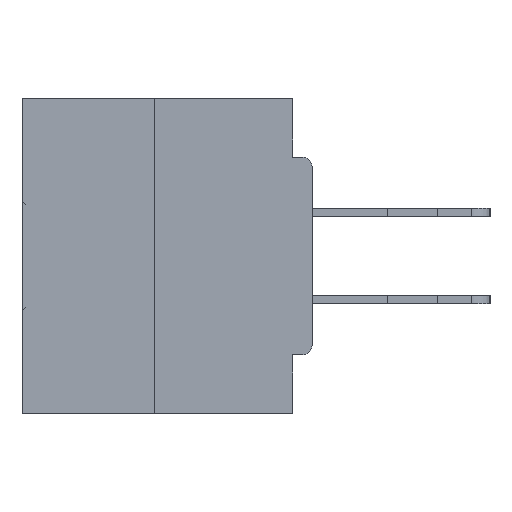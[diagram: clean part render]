
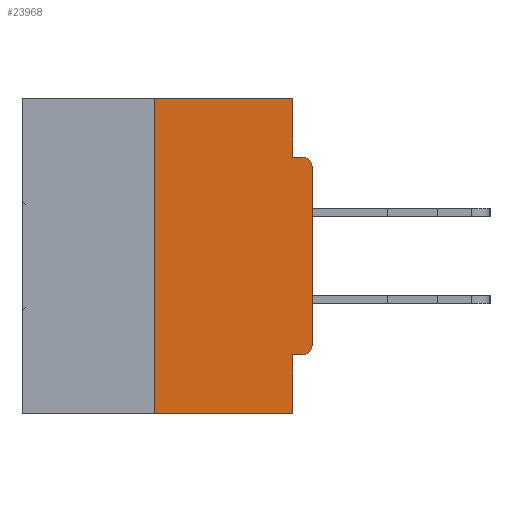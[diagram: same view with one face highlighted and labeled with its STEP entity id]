
A CAD part, left-side view. The second image highlights one B-rep face of the part: STEP entity #23968.
In plain terms, the highlighted planar face has unit normal (-1, 0, 0).
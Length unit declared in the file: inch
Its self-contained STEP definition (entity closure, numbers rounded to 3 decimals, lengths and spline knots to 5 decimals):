
#70 = CARTESIAN_POINT ( 'NONE',  ( 0., 0.015, -0.1085 ) ) ;
#123 = LINE ( 'NONE', #26899, #35440 ) ;
#1087 = VERTEX_POINT ( 'NONE', #8776 ) ;
#1341 = ORIENTED_EDGE ( 'NONE', *, *, #15577, .F. ) ;
#2043 = LINE ( 'NONE', #12261, #20298 ) ;
#2280 = EDGE_CURVE ( 'NONE', #7805, #30325, #18737, .T. ) ;
#2711 = DIRECTION ( 'NONE',  ( 0., 0., 1. ) ) ;
#2891 = LINE ( 'NONE', #3313, #11492 ) ;
#3052 = EDGE_CURVE ( 'NONE', #33925, #22421, #33907, .T. ) ;
#3313 = CARTESIAN_POINT ( 'NONE',  ( 0., 0.46, 0. ) ) ;
#4376 = VECTOR ( 'NONE', #14509, 39.37008 ) ;
#4506 = CARTESIAN_POINT ( 'NONE',  ( 0., 0.25, 0. ) ) ;
#5059 = EDGE_CURVE ( 'NONE', #30719, #29410, #36116, .T. ) ;
#5201 = VECTOR ( 'NONE', #11336, 39.37008 ) ;
#6873 = CARTESIAN_POINT ( 'NONE',  ( 0., 0.015, -0.0935 ) ) ;
#7344 = ORIENTED_EDGE ( 'NONE', *, *, #41202, .F. ) ;
#7805 = VERTEX_POINT ( 'NONE', #12624 ) ;
#8361 = DIRECTION ( 'NONE',  ( 0., 0., -1. ) ) ;
#8721 = CARTESIAN_POINT ( 'NONE',  ( 0., 0., -0.0935 ) ) ;
#8776 = CARTESIAN_POINT ( 'NONE',  ( 0., 0.031, 0. ) ) ;
#9015 = DIRECTION ( 'NONE',  ( -1., 0., 0. ) ) ;
#9055 = CARTESIAN_POINT ( 'NONE',  ( 0., 0., -0.1085 ) ) ;
#9885 = ORIENTED_EDGE ( 'NONE', *, *, #34799, .T. ) ;
#10017 = VERTEX_POINT ( 'NONE', #4506 ) ;
#10752 = VERTEX_POINT ( 'NONE', #9055 ) ;
#11336 = DIRECTION ( 'NONE',  ( 0., -1., 0. ) ) ;
#11492 = VECTOR ( 'NONE', #39909, 39.37008 ) ;
#11627 = DIRECTION ( 'NONE',  ( -1., 0., 0. ) ) ;
#12080 = CARTESIAN_POINT ( 'NONE',  ( 0., 0.25, 0. ) ) ;
#12261 = CARTESIAN_POINT ( 'NONE',  ( 0., 0., -0.4065 ) ) ;
#12624 = CARTESIAN_POINT ( 'NONE',  ( 0., 0.031, -0.0935 ) ) ;
#12968 = DIRECTION ( 'NONE',  ( 0., 0., -1. ) ) ;
#13441 = ORIENTED_EDGE ( 'NONE', *, *, #5059, .T. ) ;
#13727 = EDGE_CURVE ( 'NONE', #41756, #29410, #24661, .T. ) ;
#14509 = DIRECTION ( 'NONE',  ( 0., 0., 1. ) ) ;
#14724 = CARTESIAN_POINT ( 'NONE',  ( 0., 0., 0. ) ) ;
#14900 = CARTESIAN_POINT ( 'NONE',  ( 0., 0.015, -0.3915 ) ) ;
#15320 = DIRECTION ( 'NONE',  ( 0., 1., 0. ) ) ;
#15577 = EDGE_CURVE ( 'NONE', #1087, #7805, #123, .T. ) ;
#16372 = CARTESIAN_POINT ( 'NONE',  ( 0., 0.031, -0.4065 ) ) ;
#16711 = LINE ( 'NONE', #14724, #4376 ) ;
#16902 = AXIS2_PLACEMENT_3D ( 'NONE', #70, #9015, #30112 ) ;
#17623 = EDGE_CURVE ( 'NONE', #10752, #30325, #25954, .T. ) ;
#17891 = ORIENTED_EDGE ( 'NONE', *, *, #13727, .F. ) ;
#18737 = LINE ( 'NONE', #8721, #5201 ) ;
#19232 = ORIENTED_EDGE ( 'NONE', *, *, #3052, .T. ) ;
#19343 = EDGE_CURVE ( 'NONE', #10017, #1087, #2891, .T. ) ;
#20298 = VECTOR ( 'NONE', #15320, 39.37008 ) ;
#21587 = FACE_OUTER_BOUND ( 'NONE', #33584, .T. ) ;
#21800 = DIRECTION ( 'NONE',  ( 0., 0., -1. ) ) ;
#22421 = VERTEX_POINT ( 'NONE', #42046 ) ;
#22875 = CARTESIAN_POINT ( 'NONE',  ( 0., 0.46, 0. ) ) ;
#23968 = ADVANCED_FACE ( 'NONE', ( #21587 ), #32689, .F. ) ;
#24661 = LINE ( 'NONE', #37962, #29451 ) ;
#25738 = DIRECTION ( 'NONE',  ( 1., 0., 0. ) ) ;
#25954 = CIRCLE ( 'NONE', #16902, 0.015 ) ;
#26320 = DIRECTION ( 'NONE',  ( 0., -1., 0. ) ) ;
#26899 = CARTESIAN_POINT ( 'NONE',  ( 0., 0.031, 0. ) ) ;
#27464 = VECTOR ( 'NONE', #2711, 39.37008 ) ;
#27690 = CARTESIAN_POINT ( 'NONE',  ( 0., 0.25, -0.5 ) ) ;
#27930 = AXIS2_PLACEMENT_3D ( 'NONE', #22875, #25738, #35752 ) ;
#29062 = LINE ( 'NONE', #12080, #27464 ) ;
#29410 = VERTEX_POINT ( 'NONE', #32285 ) ;
#29451 = VECTOR ( 'NONE', #21800, 39.37008 ) ;
#29796 = CARTESIAN_POINT ( 'NONE',  ( 0., 0.46, -0.5 ) ) ;
#30112 = DIRECTION ( 'NONE',  ( 0., 0., -1. ) ) ;
#30140 = CARTESIAN_POINT ( 'NONE',  ( 0., 0.015, -0.4065 ) ) ;
#30325 = VERTEX_POINT ( 'NONE', #6873 ) ;
#30719 = VERTEX_POINT ( 'NONE', #27690 ) ;
#32127 = VECTOR ( 'NONE', #26320, 39.37008 ) ;
#32285 = CARTESIAN_POINT ( 'NONE',  ( 0., 0.031, -0.5 ) ) ;
#32422 = ORIENTED_EDGE ( 'NONE', *, *, #17623, .T. ) ;
#32689 = PLANE ( 'NONE',  #27930 ) ;
#33584 = EDGE_LOOP ( 'NONE', ( #41730, #7344, #13441, #17891, #38287, #19232, #9885, #32422, #39816, #1341 ) ) ;
#33907 = CIRCLE ( 'NONE', #40204, 0.015 ) ;
#33925 = VERTEX_POINT ( 'NONE', #30140 ) ;
#34201 = EDGE_CURVE ( 'NONE', #33925, #41756, #2043, .T. ) ;
#34799 = EDGE_CURVE ( 'NONE', #22421, #10752, #16711, .T. ) ;
#35440 = VECTOR ( 'NONE', #12968, 39.37008 ) ;
#35752 = DIRECTION ( 'NONE',  ( 0., 0., -1. ) ) ;
#36116 = LINE ( 'NONE', #29796, #32127 ) ;
#37962 = CARTESIAN_POINT ( 'NONE',  ( 0., 0.031, -0.5 ) ) ;
#38287 = ORIENTED_EDGE ( 'NONE', *, *, #34201, .F. ) ;
#39816 = ORIENTED_EDGE ( 'NONE', *, *, #2280, .F. ) ;
#39909 = DIRECTION ( 'NONE',  ( 0., -1., 0. ) ) ;
#40204 = AXIS2_PLACEMENT_3D ( 'NONE', #14900, #11627, #8361 ) ;
#41202 = EDGE_CURVE ( 'NONE', #30719, #10017, #29062, .T. ) ;
#41730 = ORIENTED_EDGE ( 'NONE', *, *, #19343, .F. ) ;
#41756 = VERTEX_POINT ( 'NONE', #16372 ) ;
#42046 = CARTESIAN_POINT ( 'NONE',  ( 0., 0., -0.3915 ) ) ;
